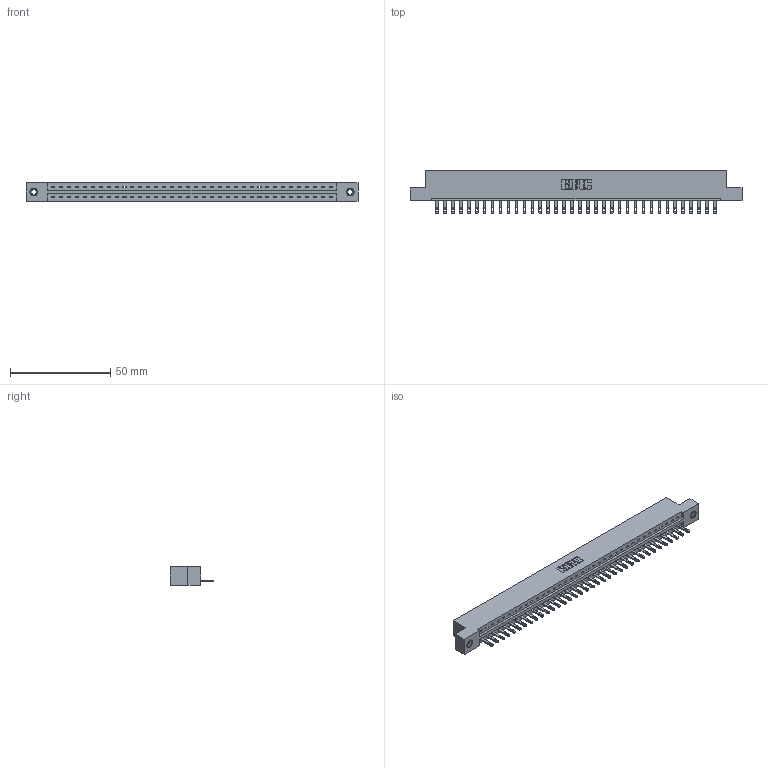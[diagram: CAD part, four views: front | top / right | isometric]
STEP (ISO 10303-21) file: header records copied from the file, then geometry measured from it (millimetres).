
FILE_DESCRIPTION (( 'STEP AP203' ), '1' );
FILE_NAME ('337-036-500-108.STEP', '2018-08-07T21:21:14', ( '' ), ( '' ), 'SwSTEP 2.0', 'SolidWorks 2016', '' );
FILE_SCHEMA (( 'CONFIG_CONTROL_DESIGN' ));
Length unit declared in the file: inch
Products named in the file (4): 337-036-500-108; 337 Part_Flush Mounting Lugs - 0.156 Dia-TI; 345-292-001_345-293-100; 345-250-001_345-250-003-102
Assembly tree (39 placements, depth 2):
  337-036-500-108
    337 Part_Flush Mounting Lugs - 0.156 Dia-TI
    345-292-001_345-293-100  x36
    345-250-001_345-250-003-102  x2
Bounding box: 165.66 x 21.85 x 9.4 mm (x, y, z)
Volume: 17158.1 mm3; surface area: 17810.9 mm2
Topology: 39 solids, 39 shells, 2262 faces, 6927 edges, 4610 vertices
Faces by surface type: plane 1542, cylinder 704, cone 12, torus 4
Entity records: 28652 total; most frequent: CARTESIAN_POINT 4969, ORIENTED_EDGE 4934, DIRECTION 4229, EDGE_CURVE 2467, LINE 2315, VECTOR 2315, VERTEX_POINT 1640, AXIS2_PLACEMENT_3D 957
